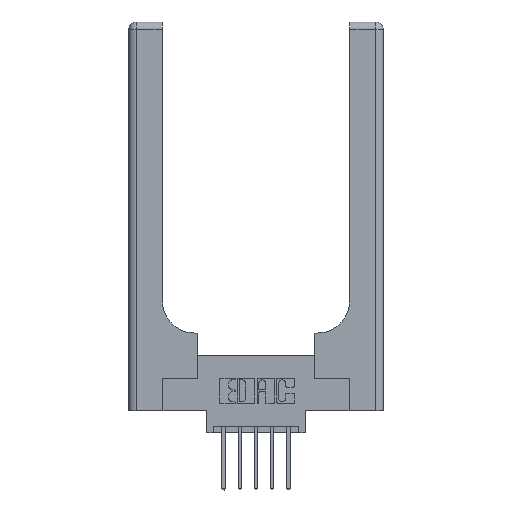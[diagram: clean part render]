
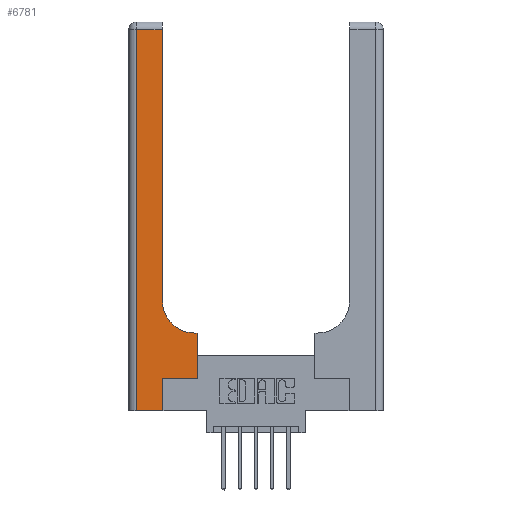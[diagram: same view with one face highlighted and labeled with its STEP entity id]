
A CAD part, top view. The second image highlights one B-rep face of the part: STEP entity #6781.
In plain terms, the highlighted planar face has unit normal (0, 0, 1).
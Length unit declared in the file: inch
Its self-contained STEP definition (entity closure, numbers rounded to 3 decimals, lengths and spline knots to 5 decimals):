
#208 = CARTESIAN_POINT ( 'NONE',  ( 0., 3., 0.37 ) ) ;
#294 = VECTOR ( 'NONE', #910, 39.37008 ) ;
#360 = CARTESIAN_POINT ( 'NONE',  ( 0.528, 0.25, 0.37 ) ) ;
#472 = ORIENTED_EDGE ( 'NONE', *, *, #12960, .T. ) ;
#690 = EDGE_CURVE ( 'NONE', #1507, #11473, #10345, .T. ) ;
#723 = LINE ( 'NONE', #12451, #3205 ) ;
#805 = EDGE_CURVE ( 'NONE', #11473, #8251, #9042, .T. ) ;
#815 = EDGE_CURVE ( 'NONE', #5129, #5873, #3435, .T. ) ;
#910 = DIRECTION ( 'NONE',  ( 0., -1., 0. ) ) ;
#971 = DIRECTION ( 'NONE',  ( 0., 1., 0. ) ) ;
#1037 = VERTEX_POINT ( 'NONE', #1376 ) ;
#1282 = DIRECTION ( 'NONE',  ( 0., 0., -1. ) ) ;
#1376 = CARTESIAN_POINT ( 'NONE',  ( 0.26, 0.85, 0.37 ) ) ;
#1507 = VERTEX_POINT ( 'NONE', #5352 ) ;
#1829 = ORIENTED_EDGE ( 'NONE', *, *, #11016, .T. ) ;
#2237 = CIRCLE ( 'NONE', #3171, 0.25 ) ;
#2238 = CARTESIAN_POINT ( 'NONE',  ( 0., 0., 0.37 ) ) ;
#2297 = VERTEX_POINT ( 'NONE', #5184 ) ;
#2893 = VERTEX_POINT ( 'NONE', #5263 ) ;
#2991 = CARTESIAN_POINT ( 'NONE',  ( 0.528, 0.25, 0.37 ) ) ;
#3029 = EDGE_CURVE ( 'NONE', #8251, #2893, #723, .T. ) ;
#3050 = LINE ( 'NONE', #7311, #11077 ) ;
#3171 = AXIS2_PLACEMENT_3D ( 'NONE', #5841, #13107, #6894 ) ;
#3204 = VERTEX_POINT ( 'NONE', #3406 ) ;
#3205 = VECTOR ( 'NONE', #10391, 39.37008 ) ;
#3406 = CARTESIAN_POINT ( 'NONE',  ( 0.26, 2.94, 0.37 ) ) ;
#3435 = LINE ( 'NONE', #4055, #294 ) ;
#3795 = EDGE_CURVE ( 'NONE', #5873, #2297, #9195, .T. ) ;
#3867 = DIRECTION ( 'NONE',  ( 1., 0., 0. ) ) ;
#4055 = CARTESIAN_POINT ( 'NONE',  ( 0.06, 3., 0.37 ) ) ;
#4102 = ORIENTED_EDGE ( 'NONE', *, *, #805, .T. ) ;
#4775 = VECTOR ( 'NONE', #3867, 39.37008 ) ;
#4839 = CARTESIAN_POINT ( 'NONE',  ( 0., 2.94, 0.37 ) ) ;
#4931 = VECTOR ( 'NONE', #7033, 39.37008 ) ;
#5129 = VERTEX_POINT ( 'NONE', #13081 ) ;
#5138 = DIRECTION ( 'NONE',  ( 0., 1., 0. ) ) ;
#5161 = EDGE_CURVE ( 'NONE', #3204, #5129, #5220, .T. ) ;
#5184 = CARTESIAN_POINT ( 'NONE',  ( 0.265, 0., 0.37 ) ) ;
#5220 = LINE ( 'NONE', #4839, #13192 ) ;
#5263 = CARTESIAN_POINT ( 'NONE',  ( 0.51, 0.6, 0.37 ) ) ;
#5352 = CARTESIAN_POINT ( 'NONE',  ( 0.265, 0.25, 0.37 ) ) ;
#5841 = CARTESIAN_POINT ( 'NONE',  ( 0.51, 0.85, 0.37 ) ) ;
#5873 = VERTEX_POINT ( 'NONE', #13229 ) ;
#5905 = DIRECTION ( 'NONE',  ( -1., 0., 0. ) ) ;
#5924 = VECTOR ( 'NONE', #5138, 39.37008 ) ;
#5982 = CARTESIAN_POINT ( 'NONE',  ( 0.26, 3., 0.37 ) ) ;
#6336 = FACE_OUTER_BOUND ( 'NONE', #9887, .T. ) ;
#6422 = VECTOR ( 'NONE', #8567, 39.37008 ) ;
#6553 = PLANE ( 'NONE',  #8598 ) ;
#6781 = ADVANCED_FACE ( 'NONE', ( #6336 ), #6553, .F. ) ;
#6894 = DIRECTION ( 'NONE',  ( 1., 0., 0. ) ) ;
#7033 = DIRECTION ( 'NONE',  ( 0., 1., 0. ) ) ;
#7311 = CARTESIAN_POINT ( 'NONE',  ( 0.265, 0., 0.37 ) ) ;
#8174 = ORIENTED_EDGE ( 'NONE', *, *, #3795, .T. ) ;
#8251 = VERTEX_POINT ( 'NONE', #13591 ) ;
#8567 = DIRECTION ( 'NONE',  ( 1., 0., 0. ) ) ;
#8598 = AXIS2_PLACEMENT_3D ( 'NONE', #208, #1282, #8657 ) ;
#8657 = DIRECTION ( 'NONE',  ( -1., 0., 0. ) ) ;
#9042 = LINE ( 'NONE', #2991, #5924 ) ;
#9195 = LINE ( 'NONE', #2238, #6422 ) ;
#9591 = ORIENTED_EDGE ( 'NONE', *, *, #690, .T. ) ;
#9773 = ORIENTED_EDGE ( 'NONE', *, *, #10159, .T. ) ;
#9887 = EDGE_LOOP ( 'NONE', ( #1829, #11096, #13593, #8174, #472, #9591, #4102, #12785, #9773 ) ) ;
#10157 = CARTESIAN_POINT ( 'NONE',  ( 0.265, 0.25, 0.37 ) ) ;
#10159 = EDGE_CURVE ( 'NONE', #2893, #1037, #2237, .T. ) ;
#10345 = LINE ( 'NONE', #10157, #4775 ) ;
#10391 = DIRECTION ( 'NONE',  ( -1., 0., 0. ) ) ;
#11016 = EDGE_CURVE ( 'NONE', #1037, #3204, #13241, .T. ) ;
#11077 = VECTOR ( 'NONE', #971, 39.37008 ) ;
#11096 = ORIENTED_EDGE ( 'NONE', *, *, #5161, .T. ) ;
#11473 = VERTEX_POINT ( 'NONE', #360 ) ;
#12451 = CARTESIAN_POINT ( 'NONE',  ( 0.26, 0.6, 0.37 ) ) ;
#12785 = ORIENTED_EDGE ( 'NONE', *, *, #3029, .T. ) ;
#12960 = EDGE_CURVE ( 'NONE', #2297, #1507, #3050, .T. ) ;
#13081 = CARTESIAN_POINT ( 'NONE',  ( 0.06, 2.94, 0.37 ) ) ;
#13107 = DIRECTION ( 'NONE',  ( 0., 0., -1. ) ) ;
#13192 = VECTOR ( 'NONE', #5905, 39.37008 ) ;
#13229 = CARTESIAN_POINT ( 'NONE',  ( 0.06, 0., 0.37 ) ) ;
#13241 = LINE ( 'NONE', #5982, #4931 ) ;
#13591 = CARTESIAN_POINT ( 'NONE',  ( 0.528, 0.6, 0.37 ) ) ;
#13593 = ORIENTED_EDGE ( 'NONE', *, *, #815, .T. ) ;
